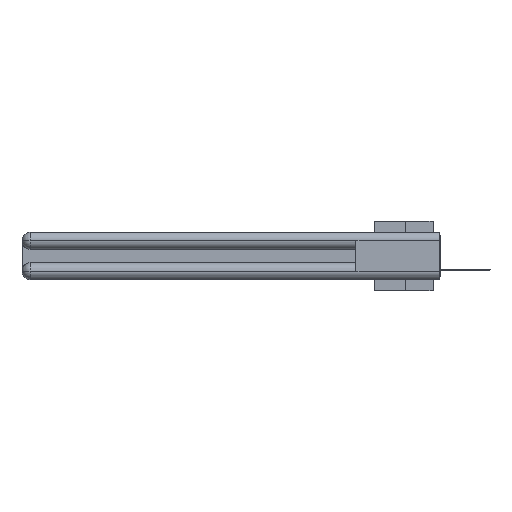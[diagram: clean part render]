
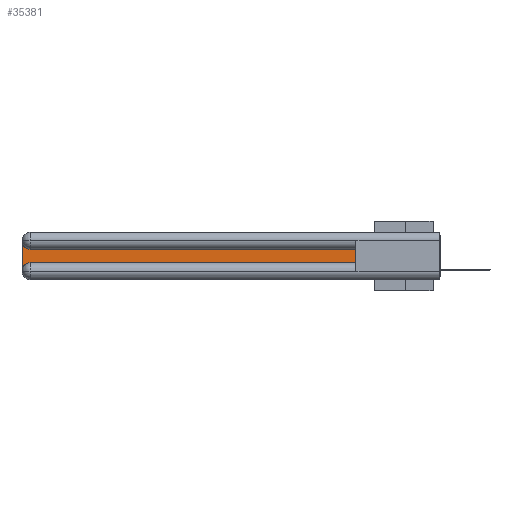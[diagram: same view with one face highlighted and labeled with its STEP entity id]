
A CAD part, left-side view. The second image highlights one B-rep face of the part: STEP entity #35381.
In plain terms, the highlighted planar face has unit normal (-1, 0, 0).
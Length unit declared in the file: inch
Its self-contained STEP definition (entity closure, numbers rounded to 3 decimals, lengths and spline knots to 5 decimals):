
#199 = CARTESIAN_POINT ( 'NONE',  ( 0.075, 0.6, -0.2175 ) ) ;
#505 = VERTEX_POINT ( 'NONE', #33621 ) ;
#1324 = EDGE_CURVE ( 'NONE', #23458, #18829, #9489, .T. ) ;
#1876 = AXIS2_PLACEMENT_3D ( 'NONE', #15936, #27829, #13008 ) ;
#2555 = DIRECTION ( 'NONE',  ( 0., 0., -1. ) ) ;
#4368 = EDGE_LOOP ( 'NONE', ( #23882, #5519, #34765, #25648, #11540, #24532 ) ) ;
#5505 = DIRECTION ( 'NONE',  ( 1., 0., 0. ) ) ;
#5519 = ORIENTED_EDGE ( 'NONE', *, *, #22556, .T. ) ;
#6774 = EDGE_CURVE ( 'NONE', #9694, #33895, #38313, .T. ) ;
#8429 = CARTESIAN_POINT ( 'NONE',  ( 0.075, 3., -0.1225 ) ) ;
#9177 = VECTOR ( 'NONE', #10677, 39.37008 ) ;
#9221 = DIRECTION ( 'NONE',  ( 0., 0., 1. ) ) ;
#9489 = LINE ( 'NONE', #10065, #32765 ) ;
#9694 = VERTEX_POINT ( 'NONE', #17367 ) ;
#10034 = EDGE_CURVE ( 'NONE', #505, #9694, #25708, .T. ) ;
#10065 = CARTESIAN_POINT ( 'NONE',  ( 0.075, 3., -0.2175 ) ) ;
#10208 = CARTESIAN_POINT ( 'NONE',  ( 0.075, 3., -0.0625 ) ) ;
#10677 = DIRECTION ( 'NONE',  ( 0., -1., 0. ) ) ;
#10729 = CARTESIAN_POINT ( 'NONE',  ( 0.075, 0.6, -0.1225 ) ) ;
#11367 = FACE_OUTER_BOUND ( 'NONE', #4368, .T. ) ;
#11540 = ORIENTED_EDGE ( 'NONE', *, *, #10034, .T. ) ;
#12556 = CARTESIAN_POINT ( 'NONE',  ( 0.075, 2.94, -0.2775 ) ) ;
#13008 = DIRECTION ( 'NONE',  ( 0., 0., -1. ) ) ;
#14063 = DIRECTION ( 'NONE',  ( 0., 1., 0. ) ) ;
#15936 = CARTESIAN_POINT ( 'NONE',  ( 0.075, 2.94, -0.0625 ) ) ;
#17367 = CARTESIAN_POINT ( 'NONE',  ( 0.075, 0.6, -0.2175 ) ) ;
#18669 = EDGE_CURVE ( 'NONE', #33895, #26560, #31246, .T. ) ;
#18745 = CIRCLE ( 'NONE', #1876, 0.06 ) ;
#18829 = VERTEX_POINT ( 'NONE', #38075 ) ;
#19857 = AXIS2_PLACEMENT_3D ( 'NONE', #8429, #5505, #2555 ) ;
#21979 = DIRECTION ( 'NONE',  ( 0., 0., -1. ) ) ;
#22556 = EDGE_CURVE ( 'NONE', #26560, #23458, #18745, .T. ) ;
#22761 = VECTOR ( 'NONE', #9221, 39.37008 ) ;
#22808 = CIRCLE ( 'NONE', #36514, 0.06 ) ;
#23458 = VERTEX_POINT ( 'NONE', #10208 ) ;
#23882 = ORIENTED_EDGE ( 'NONE', *, *, #18669, .T. ) ;
#24532 = ORIENTED_EDGE ( 'NONE', *, *, #6774, .T. ) ;
#25648 = ORIENTED_EDGE ( 'NONE', *, *, #28997, .T. ) ;
#25708 = LINE ( 'NONE', #28835, #9177 ) ;
#26219 = PLANE ( 'NONE',  #19857 ) ;
#26560 = VERTEX_POINT ( 'NONE', #27331 ) ;
#27331 = CARTESIAN_POINT ( 'NONE',  ( 0.075, 2.94, -0.1225 ) ) ;
#27829 = DIRECTION ( 'NONE',  ( 1., 0., 0. ) ) ;
#28835 = CARTESIAN_POINT ( 'NONE',  ( 0.075, 0.6, -0.2175 ) ) ;
#28997 = EDGE_CURVE ( 'NONE', #18829, #505, #22808, .T. ) ;
#31246 = LINE ( 'NONE', #10729, #33673 ) ;
#32765 = VECTOR ( 'NONE', #21979, 39.37008 ) ;
#33621 = CARTESIAN_POINT ( 'NONE',  ( 0.075, 2.94, -0.2175 ) ) ;
#33673 = VECTOR ( 'NONE', #14063, 39.37008 ) ;
#33895 = VERTEX_POINT ( 'NONE', #37530 ) ;
#34765 = ORIENTED_EDGE ( 'NONE', *, *, #1324, .T. ) ;
#35381 = ADVANCED_FACE ( 'NONE', ( #11367 ), #26219, .F. ) ;
#36514 = AXIS2_PLACEMENT_3D ( 'NONE', #12556, #37494, #37303 ) ;
#37303 = DIRECTION ( 'NONE',  ( 0., 0., -1. ) ) ;
#37494 = DIRECTION ( 'NONE',  ( 1., 0., 0. ) ) ;
#37530 = CARTESIAN_POINT ( 'NONE',  ( 0.075, 0.6, -0.1225 ) ) ;
#38075 = CARTESIAN_POINT ( 'NONE',  ( 0.075, 3., -0.2775 ) ) ;
#38313 = LINE ( 'NONE', #199, #22761 ) ;
